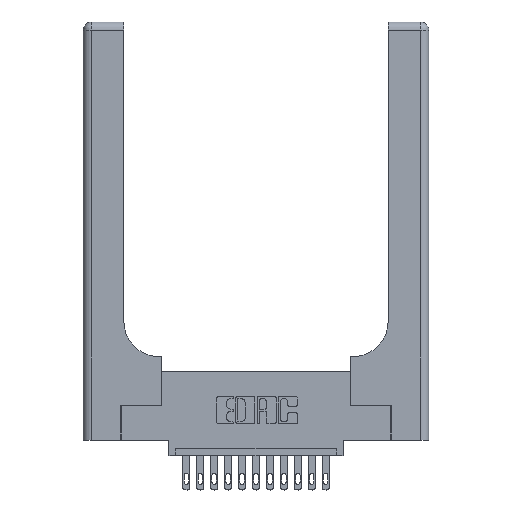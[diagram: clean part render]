
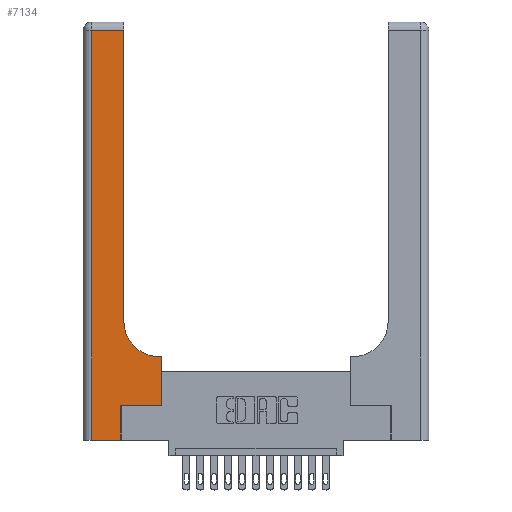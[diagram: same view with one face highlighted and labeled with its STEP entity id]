
A CAD part, top view. The second image highlights one B-rep face of the part: STEP entity #7134.
In plain terms, the highlighted planar face has unit normal (0, 0, 1).
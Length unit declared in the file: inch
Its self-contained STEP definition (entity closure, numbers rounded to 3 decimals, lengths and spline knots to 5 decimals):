
#119 = DIRECTION ( 'NONE',  ( 0., 1., 0. ) ) ;
#788 = EDGE_CURVE ( 'NONE', #11361, #11913, #12297, .T. ) ;
#1031 = CARTESIAN_POINT ( 'NONE',  ( 0., 2.94, 0.37 ) ) ;
#1194 = PLANE ( 'NONE',  #5425 ) ;
#1335 = VERTEX_POINT ( 'NONE', #9777 ) ;
#1440 = CARTESIAN_POINT ( 'NONE',  ( 0.06, 3., 0.37 ) ) ;
#1706 = VERTEX_POINT ( 'NONE', #17093 ) ;
#1772 = DIRECTION ( 'NONE',  ( 0., 1., 0. ) ) ;
#2460 = EDGE_CURVE ( 'NONE', #4434, #1706, #3265, .T. ) ;
#2578 = CARTESIAN_POINT ( 'NONE',  ( 0.269, 0., 0.37 ) ) ;
#2621 = DIRECTION ( 'NONE',  ( 0., 1., 0. ) ) ;
#2980 = VERTEX_POINT ( 'NONE', #13745 ) ;
#2981 = LINE ( 'NONE', #4819, #14474 ) ;
#3116 = VECTOR ( 'NONE', #4099, 39.37008 ) ;
#3265 = LINE ( 'NONE', #4232, #17350 ) ;
#3280 = EDGE_CURVE ( 'NONE', #14414, #5667, #3925, .T. ) ;
#3925 = LINE ( 'NONE', #5862, #12231 ) ;
#4099 = DIRECTION ( 'NONE',  ( 0., -1., 0. ) ) ;
#4114 = DIRECTION ( 'NONE',  ( -1., 0., 0. ) ) ;
#4159 = ORIENTED_EDGE ( 'NONE', *, *, #15629, .T. ) ;
#4232 = CARTESIAN_POINT ( 'NONE',  ( 0.2915, 3., 0.37 ) ) ;
#4434 = VERTEX_POINT ( 'NONE', #13911 ) ;
#4819 = CARTESIAN_POINT ( 'NONE',  ( 0.269, 0.25, 0.37 ) ) ;
#4858 = LINE ( 'NONE', #1440, #3116 ) ;
#4980 = ORIENTED_EDGE ( 'NONE', *, *, #6774, .T. ) ;
#5181 = CARTESIAN_POINT ( 'NONE',  ( 0., 0., 0.37 ) ) ;
#5278 = DIRECTION ( 'NONE',  ( 0., 0., -1. ) ) ;
#5425 = AXIS2_PLACEMENT_3D ( 'NONE', #12124, #5278, #10820 ) ;
#5667 = VERTEX_POINT ( 'NONE', #10054 ) ;
#5862 = CARTESIAN_POINT ( 'NONE',  ( 0.5585, 0.25, 0.37 ) ) ;
#6234 = ORIENTED_EDGE ( 'NONE', *, *, #11988, .T. ) ;
#6298 = DIRECTION ( 'NONE',  ( -1., 0., 0. ) ) ;
#6774 = EDGE_CURVE ( 'NONE', #1335, #11361, #4858, .T. ) ;
#6790 = CIRCLE ( 'NONE', #9263, 0.25 ) ;
#6872 = ORIENTED_EDGE ( 'NONE', *, *, #10010, .T. ) ;
#7134 = ADVANCED_FACE ( 'NONE', ( #14624 ), #1194, .F. ) ;
#8514 = ORIENTED_EDGE ( 'NONE', *, *, #2460, .T. ) ;
#9188 = LINE ( 'NONE', #10911, #16671 ) ;
#9263 = AXIS2_PLACEMENT_3D ( 'NONE', #15801, #17181, #17068 ) ;
#9777 = CARTESIAN_POINT ( 'NONE',  ( 0.06, 2.94, 0.37 ) ) ;
#10010 = EDGE_CURVE ( 'NONE', #11913, #2980, #16890, .T. ) ;
#10054 = CARTESIAN_POINT ( 'NONE',  ( 0.5585, 0.6, 0.37 ) ) ;
#10101 = EDGE_CURVE ( 'NONE', #5667, #11807, #9188, .T. ) ;
#10476 = DIRECTION ( 'NONE',  ( 1., 0., 0. ) ) ;
#10820 = DIRECTION ( 'NONE',  ( -1., 0., 0. ) ) ;
#10911 = CARTESIAN_POINT ( 'NONE',  ( 0.2915, 0.6, 0.37 ) ) ;
#11277 = LINE ( 'NONE', #1031, #15316 ) ;
#11361 = VERTEX_POINT ( 'NONE', #16477 ) ;
#11439 = VECTOR ( 'NONE', #10476, 39.37008 ) ;
#11780 = EDGE_CURVE ( 'NONE', #11807, #4434, #6790, .T. ) ;
#11807 = VERTEX_POINT ( 'NONE', #17117 ) ;
#11888 = CARTESIAN_POINT ( 'NONE',  ( 0.5585, 0.25, 0.37 ) ) ;
#11913 = VERTEX_POINT ( 'NONE', #2578 ) ;
#11988 = EDGE_CURVE ( 'NONE', #2980, #14414, #2981, .T. ) ;
#12124 = CARTESIAN_POINT ( 'NONE',  ( 0., 3., 0.37 ) ) ;
#12231 = VECTOR ( 'NONE', #1772, 39.37008 ) ;
#12297 = LINE ( 'NONE', #5181, #11439 ) ;
#12553 = ORIENTED_EDGE ( 'NONE', *, *, #11780, .T. ) ;
#13064 = DIRECTION ( 'NONE',  ( 1., 0., 0. ) ) ;
#13745 = CARTESIAN_POINT ( 'NONE',  ( 0.269, 0.25, 0.37 ) ) ;
#13911 = CARTESIAN_POINT ( 'NONE',  ( 0.2915, 0.85, 0.37 ) ) ;
#14414 = VERTEX_POINT ( 'NONE', #11888 ) ;
#14474 = VECTOR ( 'NONE', #13064, 39.37008 ) ;
#14624 = FACE_OUTER_BOUND ( 'NONE', #15477, .T. ) ;
#14675 = ORIENTED_EDGE ( 'NONE', *, *, #3280, .T. ) ;
#14952 = ORIENTED_EDGE ( 'NONE', *, *, #788, .T. ) ;
#15316 = VECTOR ( 'NONE', #6298, 39.37008 ) ;
#15477 = EDGE_LOOP ( 'NONE', ( #8514, #4159, #4980, #14952, #6872, #6234, #14675, #17450, #12553 ) ) ;
#15629 = EDGE_CURVE ( 'NONE', #1706, #1335, #11277, .T. ) ;
#15801 = CARTESIAN_POINT ( 'NONE',  ( 0.5415, 0.85, 0.37 ) ) ;
#16244 = VECTOR ( 'NONE', #2621, 39.37008 ) ;
#16288 = CARTESIAN_POINT ( 'NONE',  ( 0.269, 0., 0.37 ) ) ;
#16477 = CARTESIAN_POINT ( 'NONE',  ( 0.06, 0., 0.37 ) ) ;
#16671 = VECTOR ( 'NONE', #4114, 39.37008 ) ;
#16890 = LINE ( 'NONE', #16288, #16244 ) ;
#17068 = DIRECTION ( 'NONE',  ( 1., 0., 0. ) ) ;
#17093 = CARTESIAN_POINT ( 'NONE',  ( 0.2915, 2.94, 0.37 ) ) ;
#17117 = CARTESIAN_POINT ( 'NONE',  ( 0.5415, 0.6, 0.37 ) ) ;
#17181 = DIRECTION ( 'NONE',  ( 0., 0., -1. ) ) ;
#17350 = VECTOR ( 'NONE', #119, 39.37008 ) ;
#17450 = ORIENTED_EDGE ( 'NONE', *, *, #10101, .T. ) ;
